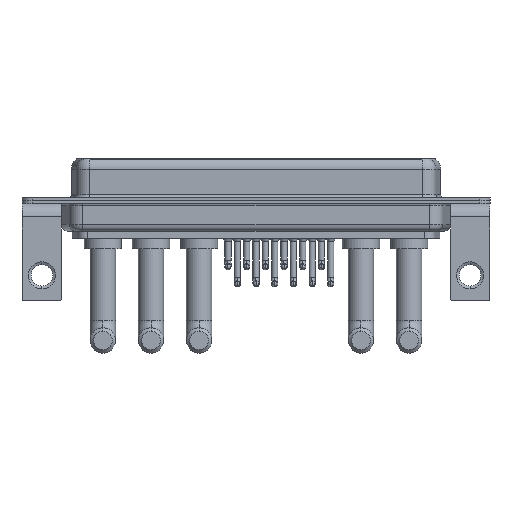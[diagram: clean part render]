
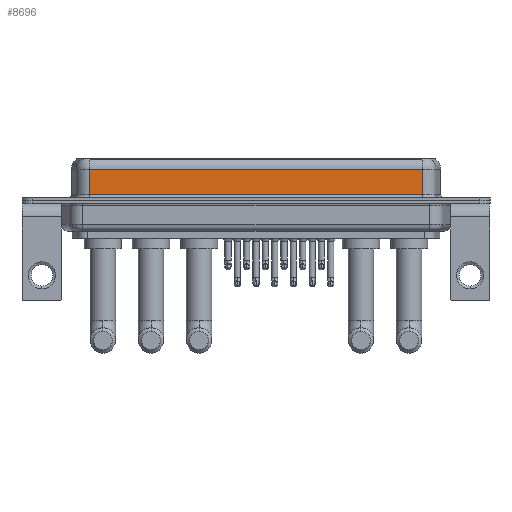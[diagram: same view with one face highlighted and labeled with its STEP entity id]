
A CAD part, front view. The second image highlights one B-rep face of the part: STEP entity #8696.
In plain terms, the highlighted planar face has unit normal (0, -1, 0).
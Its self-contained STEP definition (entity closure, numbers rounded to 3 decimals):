
#802 = EDGE_CURVE ( 'NONE', #16476, #11264, #20445, .T. ) ;
#3636 = ORIENTED_EDGE ( 'NONE', *, *, #4325, .T. ) ;
#3653 = VERTEX_POINT ( 'NONE', #12038 ) ;
#3944 = VECTOR ( 'NONE', #9324, 1000. ) ;
#4094 = CARTESIAN_POINT ( 'NONE',  ( 56.462, -3.95, 6.4 ) ) ;
#4325 = EDGE_CURVE ( 'NONE', #3653, #5727, #19401, .T. ) ;
#5727 = VERTEX_POINT ( 'NONE', #13070 ) ;
#5863 = CARTESIAN_POINT ( 'NONE',  ( 56.462, -3.95, 4.65 ) ) ;
#6782 = LINE ( 'NONE', #14642, #15810 ) ;
#8153 = DIRECTION ( 'NONE',  ( 0., 0., -1. ) ) ;
#8696 = ADVANCED_FACE ( 'NONE', ( #9044 ), #15508, .F. ) ;
#9044 = FACE_OUTER_BOUND ( 'NONE', #14925, .T. ) ;
#9324 = DIRECTION ( 'NONE',  ( -1., 0., 0. ) ) ;
#9879 = DIRECTION ( 'NONE',  ( 0., 1., 0. ) ) ;
#10045 = CARTESIAN_POINT ( 'NONE',  ( 7.038, -3.95, 6.4 ) ) ;
#11264 = VERTEX_POINT ( 'NONE', #18546 ) ;
#11364 = DIRECTION ( 'NONE',  ( 1., 0., 0. ) ) ;
#11381 = DIRECTION ( 'NONE',  ( 0., 0., 1. ) ) ;
#12038 = CARTESIAN_POINT ( 'NONE',  ( 7.038, -3.95, 4.65 ) ) ;
#12069 = EDGE_CURVE ( 'NONE', #5727, #11264, #6782, .T. ) ;
#12600 = ORIENTED_EDGE ( 'NONE', *, *, #12069, .T. ) ;
#12718 = LINE ( 'NONE', #20894, #3944 ) ;
#13040 = VECTOR ( 'NONE', #8153, 1000. ) ;
#13070 = CARTESIAN_POINT ( 'NONE',  ( 7.038, -3.95, 0.9 ) ) ;
#13396 = ORIENTED_EDGE ( 'NONE', *, *, #13666, .T. ) ;
#13666 = EDGE_CURVE ( 'NONE', #16476, #3653, #12718, .T. ) ;
#13754 = DIRECTION ( 'NONE',  ( 0., 0., -1. ) ) ;
#14520 = ORIENTED_EDGE ( 'NONE', *, *, #802, .F. ) ;
#14642 = CARTESIAN_POINT ( 'NONE',  ( 56.462, -3.95, 0.9 ) ) ;
#14925 = EDGE_LOOP ( 'NONE', ( #14520, #13396, #3636, #12600 ) ) ;
#15265 = VECTOR ( 'NONE', #13754, 1000. ) ;
#15508 = PLANE ( 'NONE',  #18403 ) ;
#15810 = VECTOR ( 'NONE', #11364, 1000. ) ;
#16476 = VERTEX_POINT ( 'NONE', #5863 ) ;
#17218 = CARTESIAN_POINT ( 'NONE',  ( 56.462, -3.95, 6.4 ) ) ;
#18403 = AXIS2_PLACEMENT_3D ( 'NONE', #17218, #9879, #11381 ) ;
#18546 = CARTESIAN_POINT ( 'NONE',  ( 56.462, -3.95, 0.9 ) ) ;
#19401 = LINE ( 'NONE', #10045, #13040 ) ;
#20445 = LINE ( 'NONE', #4094, #15265 ) ;
#20894 = CARTESIAN_POINT ( 'NONE',  ( 56.462, -3.95, 4.65 ) ) ;
